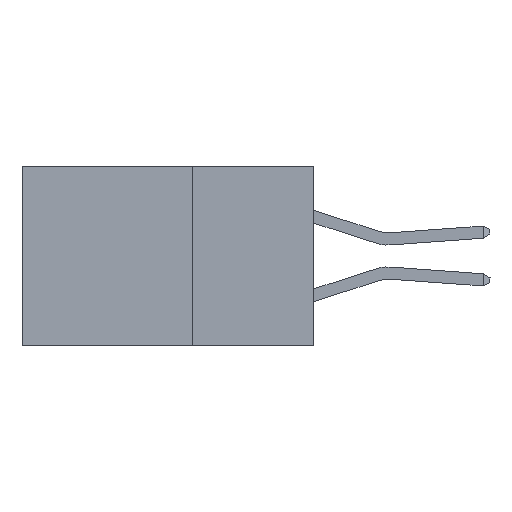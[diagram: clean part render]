
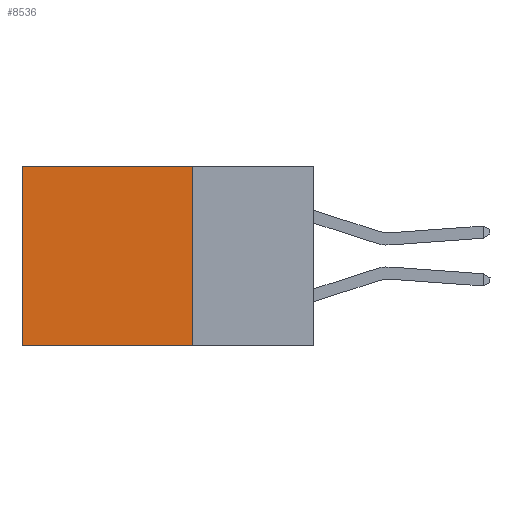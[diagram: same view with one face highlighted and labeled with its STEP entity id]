
A CAD part, left-side view. The second image highlights one B-rep face of the part: STEP entity #8536.
In plain terms, the highlighted planar face has unit normal (-1, 0, 0).
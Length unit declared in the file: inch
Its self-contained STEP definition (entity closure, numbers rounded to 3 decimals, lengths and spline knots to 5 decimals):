
#39 = LINE ( 'NONE', #13648, #25199 ) ;
#85 = VECTOR ( 'NONE', #29094, 39.37008 ) ;
#1302 = ORIENTED_EDGE ( 'NONE', *, *, #6055, .T. ) ;
#2235 = DIRECTION ( 'NONE',  ( 1., 0., 0. ) ) ;
#2576 = LINE ( 'NONE', #21529, #9362 ) ;
#6055 = EDGE_CURVE ( 'NONE', #21261, #18239, #39, .T. ) ;
#6467 = LINE ( 'NONE', #16864, #85 ) ;
#7246 = CARTESIAN_POINT ( 'NONE',  ( 0.2875, 0.6, 0. ) ) ;
#7990 = FACE_OUTER_BOUND ( 'NONE', #12442, .T. ) ;
#8536 = ADVANCED_FACE ( 'NONE', ( #7990 ), #9292, .F. ) ;
#9292 = PLANE ( 'NONE',  #28085 ) ;
#9362 = VECTOR ( 'NONE', #12169, 39.37008 ) ;
#9419 = ORIENTED_EDGE ( 'NONE', *, *, #27913, .T. ) ;
#10000 = VERTEX_POINT ( 'NONE', #25692 ) ;
#10280 = ORIENTED_EDGE ( 'NONE', *, *, #15835, .F. ) ;
#10900 = DIRECTION ( 'NONE',  ( 0., 1., 0. ) ) ;
#12169 = DIRECTION ( 'NONE',  ( 0., 1., 0. ) ) ;
#12442 = EDGE_LOOP ( 'NONE', ( #9419, #18899, #10280, #1302 ) ) ;
#13648 = CARTESIAN_POINT ( 'NONE',  ( 0.2875, 0.25, 0. ) ) ;
#14127 = CARTESIAN_POINT ( 'NONE',  ( 0.2875, 0.25, 0. ) ) ;
#14487 = DIRECTION ( 'NONE',  ( 0., 0., -1. ) ) ;
#14503 = EDGE_CURVE ( 'NONE', #15658, #10000, #2576, .T. ) ;
#15249 = CARTESIAN_POINT ( 'NONE',  ( 0.2875, 0.6, 0. ) ) ;
#15658 = VERTEX_POINT ( 'NONE', #21624 ) ;
#15835 = EDGE_CURVE ( 'NONE', #21261, #15658, #6467, .T. ) ;
#16864 = CARTESIAN_POINT ( 'NONE',  ( 0.2875, 0.25, 0. ) ) ;
#18239 = VERTEX_POINT ( 'NONE', #15249 ) ;
#18899 = ORIENTED_EDGE ( 'NONE', *, *, #14503, .F. ) ;
#19027 = VECTOR ( 'NONE', #14487, 39.37008 ) ;
#20554 = CARTESIAN_POINT ( 'NONE',  ( 0.2875, 0.25, 0. ) ) ;
#21261 = VERTEX_POINT ( 'NONE', #20554 ) ;
#21529 = CARTESIAN_POINT ( 'NONE',  ( 0.2875, 0.25, -0.37 ) ) ;
#21624 = CARTESIAN_POINT ( 'NONE',  ( 0.2875, 0.25, -0.37 ) ) ;
#22427 = LINE ( 'NONE', #7246, #19027 ) ;
#25199 = VECTOR ( 'NONE', #10900, 39.37008 ) ;
#25692 = CARTESIAN_POINT ( 'NONE',  ( 0.2875, 0.6, -0.37 ) ) ;
#27913 = EDGE_CURVE ( 'NONE', #18239, #10000, #22427, .T. ) ;
#28085 = AXIS2_PLACEMENT_3D ( 'NONE', #14127, #2235, #28597 ) ;
#28597 = DIRECTION ( 'NONE',  ( 0., 0., -1. ) ) ;
#29094 = DIRECTION ( 'NONE',  ( 0., 0., -1. ) ) ;
